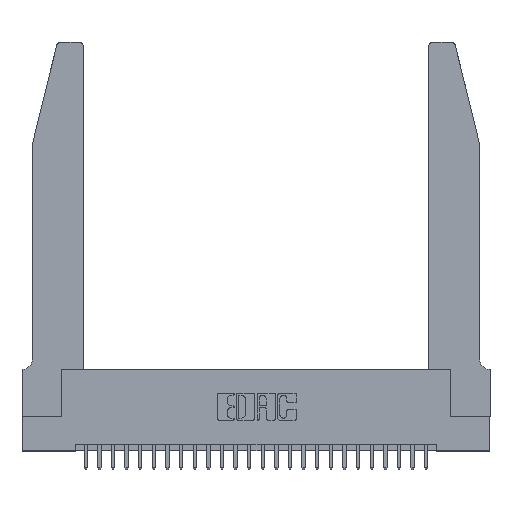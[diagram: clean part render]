
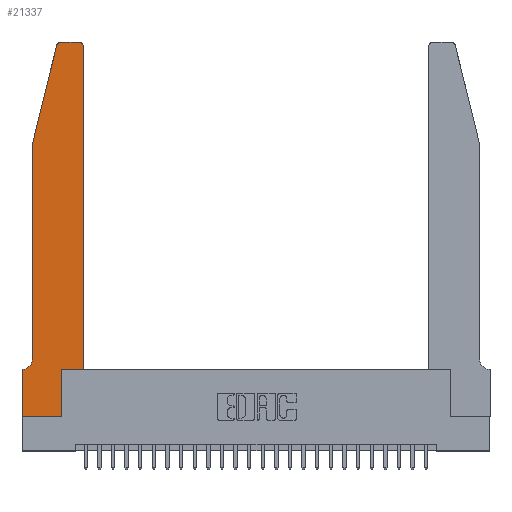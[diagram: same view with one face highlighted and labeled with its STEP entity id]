
A CAD part, top view. The second image highlights one B-rep face of the part: STEP entity #21337.
In plain terms, the highlighted planar face has unit normal (0, 0, 1).
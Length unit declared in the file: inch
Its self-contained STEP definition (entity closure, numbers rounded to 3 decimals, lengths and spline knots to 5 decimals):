
#40 = CARTESIAN_POINT ( 'NONE',  ( 0.0055, 0.42, 0.37 ) ) ;
#123 = DIRECTION ( 'NONE',  ( 0., 0., -1. ) ) ;
#149 = VECTOR ( 'NONE', #7526, 39.37008 ) ;
#263 = EDGE_CURVE ( 'NONE', #19126, #25252, #25777, .T. ) ;
#425 = EDGE_CURVE ( 'NONE', #25256, #6843, #684, .T. ) ;
#684 = LINE ( 'NONE', #24673, #16241 ) ;
#852 = DIRECTION ( 'NONE',  ( 0., 0., 1. ) ) ;
#924 = VERTEX_POINT ( 'NONE', #16254 ) ;
#2020 = VERTEX_POINT ( 'NONE', #12643 ) ;
#2057 = VERTEX_POINT ( 'NONE', #19019 ) ;
#2067 = LINE ( 'NONE', #17239, #19884 ) ;
#2269 = DIRECTION ( 'NONE',  ( -1., 0., 0. ) ) ;
#2312 = EDGE_CURVE ( 'NONE', #25252, #2057, #24705, .T. ) ;
#2485 = AXIS2_PLACEMENT_3D ( 'NONE', #40, #123, #2269 ) ;
#2588 = VERTEX_POINT ( 'NONE', #26253 ) ;
#3000 = ORIENTED_EDGE ( 'NONE', *, *, #2312, .T. ) ;
#3200 = VERTEX_POINT ( 'NONE', #22790 ) ;
#4106 = CARTESIAN_POINT ( 'NONE',  ( 0.4205, 2.75, 0.37 ) ) ;
#4331 = CIRCLE ( 'NONE', #2485, 0.07 ) ;
#4421 = DIRECTION ( 'NONE',  ( -1., 0., 0. ) ) ;
#4483 = CARTESIAN_POINT ( 'NONE',  ( 0.0755, 2., 0.37 ) ) ;
#6083 = EDGE_LOOP ( 'NONE', ( #10982, #3000, #8659, #11820, #22407, #8781, #17162, #22416, #17813, #22219, #16235, #6415 ) ) ;
#6161 = CARTESIAN_POINT ( 'NONE',  ( 0.4505, 0.35, 0.37 ) ) ;
#6218 = CARTESIAN_POINT ( 'NONE',  ( 0.2865, 0.35, 0.37 ) ) ;
#6415 = ORIENTED_EDGE ( 'NONE', *, *, #15076, .T. ) ;
#6499 = EDGE_CURVE ( 'NONE', #2020, #924, #22148, .T. ) ;
#6606 = DIRECTION ( 'NONE',  ( -1., 0., 0. ) ) ;
#6843 = VERTEX_POINT ( 'NONE', #14084 ) ;
#7054 = VECTOR ( 'NONE', #12954, 39.37008 ) ;
#7526 = DIRECTION ( 'NONE',  ( 0., 1., 0. ) ) ;
#7804 = VERTEX_POINT ( 'NONE', #19368 ) ;
#8015 = EDGE_CURVE ( 'NONE', #924, #17232, #15002, .T. ) ;
#8046 = DIRECTION ( 'NONE',  ( 0., -1., 0. ) ) ;
#8659 = ORIENTED_EDGE ( 'NONE', *, *, #20297, .T. ) ;
#8781 = ORIENTED_EDGE ( 'NONE', *, *, #20411, .T. ) ;
#9102 = AXIS2_PLACEMENT_3D ( 'NONE', #24904, #16243, #24629 ) ;
#9494 = CARTESIAN_POINT ( 'NONE',  ( 0., 0., 0.37 ) ) ;
#9739 = CARTESIAN_POINT ( 'NONE',  ( 0.4505, 0.35, 0.37 ) ) ;
#9961 = FACE_OUTER_BOUND ( 'NONE', #6083, .T. ) ;
#10103 = LINE ( 'NONE', #9739, #149 ) ;
#10133 = CARTESIAN_POINT ( 'NONE',  ( 0.0055, 0.35, 0.37 ) ) ;
#10301 = EDGE_CURVE ( 'NONE', #6843, #20116, #4331, .T. ) ;
#10420 = VECTOR ( 'NONE', #24259, 39.37008 ) ;
#10982 = ORIENTED_EDGE ( 'NONE', *, *, #263, .T. ) ;
#11280 = VECTOR ( 'NONE', #4421, 39.37008 ) ;
#11282 = CARTESIAN_POINT ( 'NONE',  ( 0.2865, 0., 0.37 ) ) ;
#11820 = ORIENTED_EDGE ( 'NONE', *, *, #425, .T. ) ;
#11877 = VECTOR ( 'NONE', #25701, 39.37008 ) ;
#12199 = CARTESIAN_POINT ( 'NONE',  ( 0., 0.35, 0.37 ) ) ;
#12303 = CARTESIAN_POINT ( 'NONE',  ( 0.284, 2.75, 0.37 ) ) ;
#12358 = EDGE_CURVE ( 'NONE', #17232, #3200, #22422, .T. ) ;
#12386 = DIRECTION ( 'NONE',  ( 0., 0., 1. ) ) ;
#12643 = CARTESIAN_POINT ( 'NONE',  ( 0., 0.35, 0.37 ) ) ;
#12649 = LINE ( 'NONE', #4483, #7054 ) ;
#12954 = DIRECTION ( 'NONE',  ( -0.239, -0.971, 0. ) ) ;
#14084 = CARTESIAN_POINT ( 'NONE',  ( 0.0755, 0.42, 0.37 ) ) ;
#15002 = LINE ( 'NONE', #9494, #10420 ) ;
#15076 = EDGE_CURVE ( 'NONE', #7804, #19126, #22617, .T. ) ;
#16235 = ORIENTED_EDGE ( 'NONE', *, *, #27007, .T. ) ;
#16241 = VECTOR ( 'NONE', #8046, 39.37008 ) ;
#16243 = DIRECTION ( 'NONE',  ( 0., 0., 1. ) ) ;
#16254 = CARTESIAN_POINT ( 'NONE',  ( 0., 0., 0.37 ) ) ;
#16369 = DIRECTION ( 'NONE',  ( 1., 0., 0. ) ) ;
#16833 = VECTOR ( 'NONE', #20345, 39.37008 ) ;
#17162 = ORIENTED_EDGE ( 'NONE', *, *, #6499, .T. ) ;
#17232 = VERTEX_POINT ( 'NONE', #11282 ) ;
#17239 = CARTESIAN_POINT ( 'NONE',  ( 0.0755, 0.35, 0.37 ) ) ;
#17813 = ORIENTED_EDGE ( 'NONE', *, *, #12358, .T. ) ;
#19019 = CARTESIAN_POINT ( 'NONE',  ( 0.25487, 2.72718, 0.37 ) ) ;
#19126 = VERTEX_POINT ( 'NONE', #4106 ) ;
#19368 = CARTESIAN_POINT ( 'NONE',  ( 0.4505, 2.72, 0.37 ) ) ;
#19884 = VECTOR ( 'NONE', #6606, 39.37008 ) ;
#20116 = VERTEX_POINT ( 'NONE', #10133 ) ;
#20297 = EDGE_CURVE ( 'NONE', #2057, #25256, #12649, .T. ) ;
#20345 = DIRECTION ( 'NONE',  ( 0., 1., 0. ) ) ;
#20411 = EDGE_CURVE ( 'NONE', #20116, #2020, #2067, .T. ) ;
#20622 = AXIS2_PLACEMENT_3D ( 'NONE', #26145, #852, #24403 ) ;
#20706 = CARTESIAN_POINT ( 'NONE',  ( 0.0755, 2., 0.37 ) ) ;
#20786 = LINE ( 'NONE', #6161, #11877 ) ;
#21337 = ADVANCED_FACE ( 'NONE', ( #9961 ), #25027, .T. ) ;
#22148 = LINE ( 'NONE', #27114, #24114 ) ;
#22219 = ORIENTED_EDGE ( 'NONE', *, *, #22434, .T. ) ;
#22407 = ORIENTED_EDGE ( 'NONE', *, *, #10301, .T. ) ;
#22416 = ORIENTED_EDGE ( 'NONE', *, *, #8015, .T. ) ;
#22422 = LINE ( 'NONE', #6218, #16833 ) ;
#22434 = EDGE_CURVE ( 'NONE', #3200, #2588, #20786, .T. ) ;
#22617 = CIRCLE ( 'NONE', #20622, 0.03 ) ;
#22790 = CARTESIAN_POINT ( 'NONE',  ( 0.2865, 0.35, 0.37 ) ) ;
#24114 = VECTOR ( 'NONE', #27292, 39.37008 ) ;
#24259 = DIRECTION ( 'NONE',  ( 1., 0., 0. ) ) ;
#24403 = DIRECTION ( 'NONE',  ( 1., 0., 0. ) ) ;
#24629 = DIRECTION ( 'NONE',  ( 1., 0., 0. ) ) ;
#24673 = CARTESIAN_POINT ( 'NONE',  ( 0.0755, 2., 0.37 ) ) ;
#24705 = CIRCLE ( 'NONE', #9102, 0.03 ) ;
#24904 = CARTESIAN_POINT ( 'NONE',  ( 0.284, 2.72, 0.37 ) ) ;
#25027 = PLANE ( 'NONE',  #27059 ) ;
#25252 = VERTEX_POINT ( 'NONE', #12303 ) ;
#25256 = VERTEX_POINT ( 'NONE', #20706 ) ;
#25452 = CARTESIAN_POINT ( 'NONE',  ( 0.2605, 2.75, 0.37 ) ) ;
#25701 = DIRECTION ( 'NONE',  ( 1., 0., 0. ) ) ;
#25777 = LINE ( 'NONE', #25452, #11280 ) ;
#26145 = CARTESIAN_POINT ( 'NONE',  ( 0.4205, 2.72, 0.37 ) ) ;
#26253 = CARTESIAN_POINT ( 'NONE',  ( 0.4505, 0.35, 0.37 ) ) ;
#27007 = EDGE_CURVE ( 'NONE', #2588, #7804, #10103, .T. ) ;
#27059 = AXIS2_PLACEMENT_3D ( 'NONE', #12199, #12386, #16369 ) ;
#27114 = CARTESIAN_POINT ( 'NONE',  ( 0., 0., 0.37 ) ) ;
#27292 = DIRECTION ( 'NONE',  ( 0., -1., 0. ) ) ;
